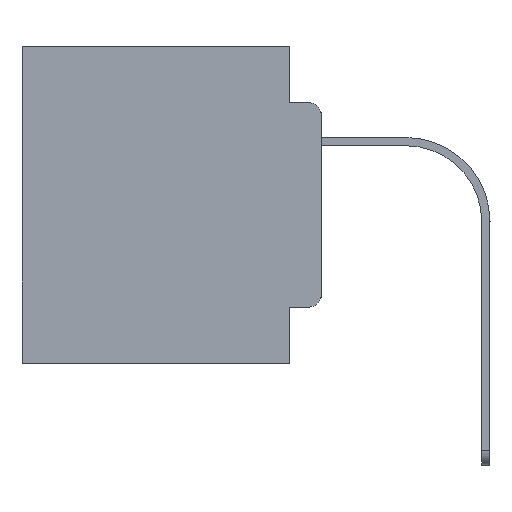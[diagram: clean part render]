
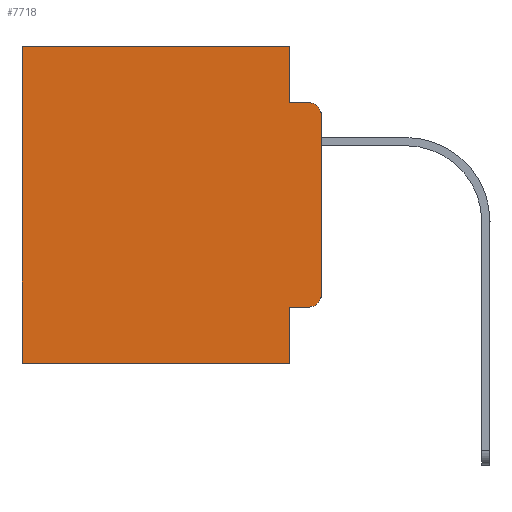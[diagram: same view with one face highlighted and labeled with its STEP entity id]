
A CAD part, left-side view. The second image highlights one B-rep face of the part: STEP entity #7718.
In plain terms, the highlighted planar face has unit normal (-1, 0, 0).
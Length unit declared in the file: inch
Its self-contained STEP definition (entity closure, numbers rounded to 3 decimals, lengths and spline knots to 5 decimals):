
#182 = CARTESIAN_POINT ( 'NONE',  ( 0.298, 0.02, -0.3915 ) ) ;
#678 = VECTOR ( 'NONE', #10761, 39.37008 ) ;
#1512 = ORIENTED_EDGE ( 'NONE', *, *, #12162, .F. ) ;
#1622 = VECTOR ( 'NONE', #6227, 39.37008 ) ;
#1672 = CARTESIAN_POINT ( 'NONE',  ( 0.298, 0., 0. ) ) ;
#1726 = DIRECTION ( 'NONE',  ( 0., 0., -1. ) ) ;
#1853 = VERTEX_POINT ( 'NONE', #10589 ) ;
#1928 = EDGE_LOOP ( 'NONE', ( #1512, #22488, #21403, #11024, #5993, #10730, #12841, #7778, #11453, #10382 ) ) ;
#1943 = CARTESIAN_POINT ( 'NONE',  ( 0.298, 0., -0.5 ) ) ;
#2149 = DIRECTION ( 'NONE',  ( 0., 0., -1. ) ) ;
#2163 = LINE ( 'NONE', #9559, #22416 ) ;
#2216 = EDGE_CURVE ( 'NONE', #11905, #10498, #2163, .T. ) ;
#2666 = CARTESIAN_POINT ( 'NONE',  ( 0.298, 0.051, 0. ) ) ;
#3038 = DIRECTION ( 'NONE',  ( 0., -1., 0. ) ) ;
#3288 = EDGE_CURVE ( 'NONE', #21758, #9570, #15156, .T. ) ;
#4056 = VECTOR ( 'NONE', #16174, 39.37008 ) ;
#4460 = VERTEX_POINT ( 'NONE', #11248 ) ;
#4740 = LINE ( 'NONE', #2666, #4843 ) ;
#4843 = VECTOR ( 'NONE', #16665, 39.37008 ) ;
#4936 = LINE ( 'NONE', #22926, #678 ) ;
#4996 = CARTESIAN_POINT ( 'NONE',  ( 0.298, 0.051, -0.0885 ) ) ;
#5126 = CARTESIAN_POINT ( 'NONE',  ( 0.298, 0.473, -0.5 ) ) ;
#5625 = VECTOR ( 'NONE', #3038, 39.37008 ) ;
#5782 = FACE_OUTER_BOUND ( 'NONE', #1928, .T. ) ;
#5993 = ORIENTED_EDGE ( 'NONE', *, *, #9115, .T. ) ;
#6227 = DIRECTION ( 'NONE',  ( 0., 0., -1. ) ) ;
#6536 = AXIS2_PLACEMENT_3D ( 'NONE', #182, #17659, #1726 ) ;
#6854 = AXIS2_PLACEMENT_3D ( 'NONE', #10661, #19696, #19317 ) ;
#7470 = VERTEX_POINT ( 'NONE', #24543 ) ;
#7516 = CARTESIAN_POINT ( 'NONE',  ( 0.298, 0., -0.1085 ) ) ;
#7718 = ADVANCED_FACE ( 'NONE', ( #5782 ), #7856, .F. ) ;
#7778 = ORIENTED_EDGE ( 'NONE', *, *, #9341, .F. ) ;
#7856 = PLANE ( 'NONE',  #17848 ) ;
#8274 = EDGE_CURVE ( 'NONE', #17997, #10632, #24646, .T. ) ;
#8555 = VECTOR ( 'NONE', #23448, 39.37008 ) ;
#8740 = EDGE_CURVE ( 'NONE', #21179, #10632, #18021, .T. ) ;
#9115 = EDGE_CURVE ( 'NONE', #1853, #21758, #4936, .T. ) ;
#9341 = EDGE_CURVE ( 'NONE', #11905, #7470, #4740, .T. ) ;
#9559 = CARTESIAN_POINT ( 'NONE',  ( 0.298, 0.051, -0.4115 ) ) ;
#9570 = VERTEX_POINT ( 'NONE', #5126 ) ;
#10382 = ORIENTED_EDGE ( 'NONE', *, *, #16275, .T. ) ;
#10498 = VERTEX_POINT ( 'NONE', #21633 ) ;
#10578 = EDGE_CURVE ( 'NONE', #7470, #9570, #21114, .T. ) ;
#10589 = CARTESIAN_POINT ( 'NONE',  ( 0.298, 0.051, 0. ) ) ;
#10628 = DIRECTION ( 'NONE',  ( 0., 0., -1. ) ) ;
#10632 = VERTEX_POINT ( 'NONE', #23698 ) ;
#10661 = CARTESIAN_POINT ( 'NONE',  ( 0.298, 0.02, -0.1085 ) ) ;
#10730 = ORIENTED_EDGE ( 'NONE', *, *, #3288, .T. ) ;
#10761 = DIRECTION ( 'NONE',  ( 0., 1., 0. ) ) ;
#11024 = ORIENTED_EDGE ( 'NONE', *, *, #16830, .F. ) ;
#11130 = VECTOR ( 'NONE', #10628, 39.37008 ) ;
#11248 = CARTESIAN_POINT ( 'NONE',  ( 0.298, 0., -0.3915 ) ) ;
#11453 = ORIENTED_EDGE ( 'NONE', *, *, #2216, .T. ) ;
#11905 = VERTEX_POINT ( 'NONE', #12815 ) ;
#12018 = CARTESIAN_POINT ( 'NONE',  ( 0.298, 0.473, 0. ) ) ;
#12162 = EDGE_CURVE ( 'NONE', #21179, #4460, #19403, .T. ) ;
#12708 = CARTESIAN_POINT ( 'NONE',  ( 0.298, 0.473, 0. ) ) ;
#12815 = CARTESIAN_POINT ( 'NONE',  ( 0.298, 0.051, -0.4115 ) ) ;
#12841 = ORIENTED_EDGE ( 'NONE', *, *, #10578, .F. ) ;
#13683 = CARTESIAN_POINT ( 'NONE',  ( 0.298, 0., 0. ) ) ;
#15156 = LINE ( 'NONE', #12708, #11130 ) ;
#16174 = DIRECTION ( 'NONE',  ( 0., 0., -1. ) ) ;
#16275 = EDGE_CURVE ( 'NONE', #10498, #4460, #17711, .T. ) ;
#16665 = DIRECTION ( 'NONE',  ( 0., 0., -1. ) ) ;
#16830 = EDGE_CURVE ( 'NONE', #1853, #17997, #23948, .T. ) ;
#17659 = DIRECTION ( 'NONE',  ( -1., 0., 0. ) ) ;
#17711 = CIRCLE ( 'NONE', #6536, 0.02 ) ;
#17832 = DIRECTION ( 'NONE',  ( 0., -1., 0. ) ) ;
#17848 = AXIS2_PLACEMENT_3D ( 'NONE', #13683, #23640, #2149 ) ;
#17997 = VERTEX_POINT ( 'NONE', #23707 ) ;
#18021 = CIRCLE ( 'NONE', #6854, 0.02 ) ;
#19317 = DIRECTION ( 'NONE',  ( 0., 0., -1. ) ) ;
#19403 = LINE ( 'NONE', #1672, #4056 ) ;
#19696 = DIRECTION ( 'NONE',  ( -1., 0., 0. ) ) ;
#21114 = LINE ( 'NONE', #1943, #8555 ) ;
#21179 = VERTEX_POINT ( 'NONE', #7516 ) ;
#21403 = ORIENTED_EDGE ( 'NONE', *, *, #8274, .F. ) ;
#21633 = CARTESIAN_POINT ( 'NONE',  ( 0.298, 0.02, -0.4115 ) ) ;
#21758 = VERTEX_POINT ( 'NONE', #12018 ) ;
#22416 = VECTOR ( 'NONE', #17832, 39.37008 ) ;
#22488 = ORIENTED_EDGE ( 'NONE', *, *, #8740, .T. ) ;
#22926 = CARTESIAN_POINT ( 'NONE',  ( 0.298, 0., 0. ) ) ;
#23448 = DIRECTION ( 'NONE',  ( 0., 1., 0. ) ) ;
#23640 = DIRECTION ( 'NONE',  ( 1., 0., 0. ) ) ;
#23698 = CARTESIAN_POINT ( 'NONE',  ( 0.298, 0.02, -0.0885 ) ) ;
#23707 = CARTESIAN_POINT ( 'NONE',  ( 0.298, 0.051, -0.0885 ) ) ;
#23948 = LINE ( 'NONE', #24077, #1622 ) ;
#24077 = CARTESIAN_POINT ( 'NONE',  ( 0.298, 0.051, 0. ) ) ;
#24543 = CARTESIAN_POINT ( 'NONE',  ( 0.298, 0.051, -0.5 ) ) ;
#24646 = LINE ( 'NONE', #4996, #5625 ) ;
